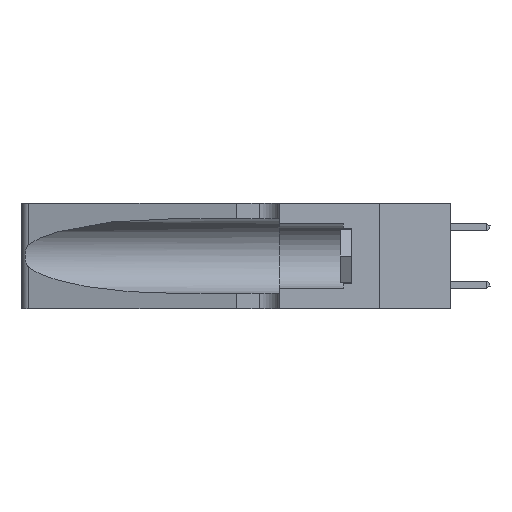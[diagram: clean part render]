
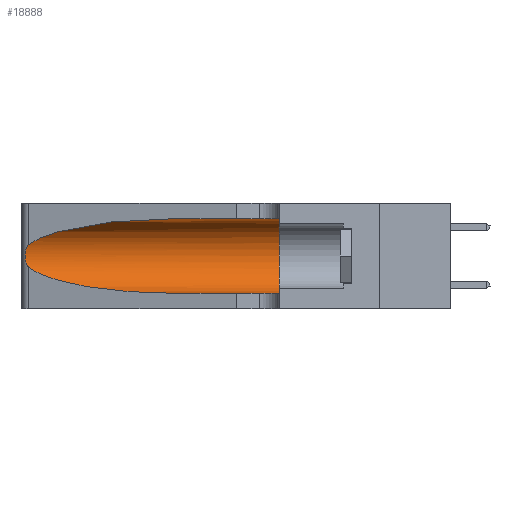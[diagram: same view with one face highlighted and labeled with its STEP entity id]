
A CAD part, left-side view. The second image highlights one B-rep face of the part: STEP entity #18888.
In plain terms, the highlighted cylindrical face has radius 3.308 mm (diameter 6.617 mm), a partial arc.
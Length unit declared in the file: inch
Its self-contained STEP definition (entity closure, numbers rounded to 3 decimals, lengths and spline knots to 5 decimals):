
#78 = CARTESIAN_POINT ( 'NONE',  ( 0.1305, 1.61858, 0.185 ) ) ;
#331 = AXIS2_PLACEMENT_3D ( 'NONE', #78, #10808, #15118 ) ;
#923 = VERTEX_POINT ( 'NONE', #23776 ) ;
#1726 = LINE ( 'NONE', #21640, #12320 ) ;
#1772 = CARTESIAN_POINT ( 'NONE',  ( 0.1305, 0.72297, 0.31525 ) ) ;
#1822 = EDGE_CURVE ( 'NONE', #23802, #9129, #22448, .T. ) ;
#2051 = CARTESIAN_POINT ( 'NONE',  ( 0.25856, 1.23593, 0.16098 ) ) ;
#2554 = CARTESIAN_POINT ( 'NONE',  ( 0.1305, 0.72297, 0.31525 ) ) ;
#3502 = ORIENTED_EDGE ( 'NONE', *, *, #5940, .T. ) ;
#3691 = CARTESIAN_POINT ( 'NONE',  ( 0.25487, 1.22718, 0.14631 ) ) ;
#4161 = CARTESIAN_POINT ( 'NONE',  ( 0.25639, 1.23186, 0.15144 ) ) ;
#5436 = CARTESIAN_POINT ( 'NONE',  ( 0.2373, 1.15595, 0.08982 ) ) ;
#5483 = LINE ( 'NONE', #10840, #10451 ) ;
#5678 = CIRCLE ( 'NONE', #11057, 0.13025 ) ;
#5940 = EDGE_CURVE ( 'NONE', #923, #23802, #12637, .T. ) ;
#6181 = VERTEX_POINT ( 'NONE', #7060 ) ;
#6287 = EDGE_CURVE ( 'NONE', #13009, #6181, #5678, .T. ) ;
#6307 = CARTESIAN_POINT ( 'NONE',  ( 0.25487, 1.22718, 0.14631 ) ) ;
#7060 = CARTESIAN_POINT ( 'NONE',  ( 0.1305, 0.35, 0.05475 ) ) ;
#8197 = CARTESIAN_POINT ( 'NONE',  ( 0.2373, 1.15595, 0.28018 ) ) ;
#8360 = CARTESIAN_POINT ( 'NONE',  ( 0.25639, 1.23184, 0.21858 ) ) ;
#8706 = FACE_OUTER_BOUND ( 'NONE', #13046, .T. ) ;
#9129 = VERTEX_POINT ( 'NONE', #16819 ) ;
#9145 = ORIENTED_EDGE ( 'NONE', *, *, #1822, .T. ) ;
#9790 = CARTESIAN_POINT ( 'NONE',  ( 0.25487, 1.22718, 0.14631 ) ) ;
#10451 = VECTOR ( 'NONE', #12997, 39.37008 ) ;
#10462 = CARTESIAN_POINT ( 'NONE',  ( 0.25854, 1.2359, 0.20912 ) ) ;
#10583 =( BOUNDED_CURVE ( )  B_SPLINE_CURVE ( 3, ( #1772, #20852, #8197, #22942 ),
 .UNSPECIFIED., .F., .F. ) 
 B_SPLINE_CURVE_WITH_KNOTS ( ( 4, 4 ),
 ( 1.5708, 2.84003 ),
 .UNSPECIFIED. ) 
 CURVE ( )  GEOMETRIC_REPRESENTATION_ITEM ( )  RATIONAL_B_SPLINE_CURVE ( ( 1., 0.87, 0.87, 1. ) ) 
 REPRESENTATION_ITEM ( '' )  );
#10808 = DIRECTION ( 'NONE',  ( 0., -1., 0. ) ) ;
#10840 = CARTESIAN_POINT ( 'NONE',  ( 0.1305, 1.61858, 0.05475 ) ) ;
#11057 = AXIS2_PLACEMENT_3D ( 'NONE', #24269, #11652, #26389 ) ;
#11652 = DIRECTION ( 'NONE',  ( 0., 1., 0. ) ) ;
#12277 = VERTEX_POINT ( 'NONE', #2554 ) ;
#12320 = VECTOR ( 'NONE', #23739, 39.37008 ) ;
#12603 = CARTESIAN_POINT ( 'NONE',  ( 0.26075, 1.23896, 0.19203 ) ) ;
#12637 = B_SPLINE_CURVE_WITH_KNOTS ( 'NONE', 3,
 ( #18894, #21031, #8360, #23122, #10462, #25224, #12603, #27333, #14761, #2051, #16870, #4161, #18993, #6307 ),
 .UNSPECIFIED., .F., .F.,
 ( 4, 2, 2, 2, 2, 2, 4 ),
 ( 0., 0.00027, 0.00053, 0.00107, 0.0016, 0.00187, 0.00214 ),
 .UNSPECIFIED. ) ;
#12997 = DIRECTION ( 'NONE',  ( 0., -1., 0. ) ) ;
#13009 = VERTEX_POINT ( 'NONE', #21774 ) ;
#13046 = EDGE_LOOP ( 'NONE', ( #14138, #3502, #9145, #26640, #16120, #22371 ) ) ;
#14138 = ORIENTED_EDGE ( 'NONE', *, *, #15998, .T. ) ;
#14761 = CARTESIAN_POINT ( 'NONE',  ( 0.26017, 1.23833, 0.17102 ) ) ;
#15118 = DIRECTION ( 'NONE',  ( 0., 0., -1. ) ) ;
#15998 = EDGE_CURVE ( 'NONE', #12277, #923, #10583, .T. ) ;
#16120 = ORIENTED_EDGE ( 'NONE', *, *, #6287, .F. ) ;
#16819 = CARTESIAN_POINT ( 'NONE',  ( 0.1305, 0.72297, 0.05475 ) ) ;
#16870 = CARTESIAN_POINT ( 'NONE',  ( 0.25789, 1.23486, 0.15765 ) ) ;
#18888 = ADVANCED_FACE ( 'NONE', ( #8706 ), #24859, .F. ) ;
#18894 = CARTESIAN_POINT ( 'NONE',  ( 0.25487, 1.22718, 0.22369 ) ) ;
#18942 = EDGE_CURVE ( 'NONE', #12277, #13009, #1726, .T. ) ;
#18993 = CARTESIAN_POINT ( 'NONE',  ( 0.25555, 1.22993, 0.14849 ) ) ;
#20346 = CARTESIAN_POINT ( 'NONE',  ( 0.18966, 0.96281, 0.05475 ) ) ;
#20852 = CARTESIAN_POINT ( 'NONE',  ( 0.18966, 0.96281, 0.31525 ) ) ;
#21031 = CARTESIAN_POINT ( 'NONE',  ( 0.25555, 1.22994, 0.2215 ) ) ;
#21640 = CARTESIAN_POINT ( 'NONE',  ( 0.1305, 1.61858, 0.31525 ) ) ;
#21774 = CARTESIAN_POINT ( 'NONE',  ( 0.1305, 0.35, 0.31525 ) ) ;
#22371 = ORIENTED_EDGE ( 'NONE', *, *, #18942, .F. ) ;
#22448 =( BOUNDED_CURVE ( )  B_SPLINE_CURVE ( 3, ( #9790, #5436, #20346, #24545 ),
 .UNSPECIFIED., .F., .T. ) 
 B_SPLINE_CURVE_WITH_KNOTS ( ( 4, 4 ),
 ( 3.44316, 4.71239 ),
 .UNSPECIFIED. ) 
 CURVE ( )  GEOMETRIC_REPRESENTATION_ITEM ( )  RATIONAL_B_SPLINE_CURVE ( ( 1., 0.87, 0.87, 1. ) ) 
 REPRESENTATION_ITEM ( '' )  );
#22942 = CARTESIAN_POINT ( 'NONE',  ( 0.25487, 1.22718, 0.22369 ) ) ;
#23122 = CARTESIAN_POINT ( 'NONE',  ( 0.25787, 1.23484, 0.2124 ) ) ;
#23346 = EDGE_CURVE ( 'NONE', #9129, #6181, #5483, .T. ) ;
#23739 = DIRECTION ( 'NONE',  ( 0., -1., 0. ) ) ;
#23776 = CARTESIAN_POINT ( 'NONE',  ( 0.25487, 1.22718, 0.22369 ) ) ;
#23802 = VERTEX_POINT ( 'NONE', #3691 ) ;
#24269 = CARTESIAN_POINT ( 'NONE',  ( 0.1305, 0.35, 0.185 ) ) ;
#24545 = CARTESIAN_POINT ( 'NONE',  ( 0.1305, 0.72297, 0.05475 ) ) ;
#24859 = CYLINDRICAL_SURFACE ( 'NONE', #331, 0.13025 ) ;
#25224 = CARTESIAN_POINT ( 'NONE',  ( 0.26018, 1.23835, 0.19895 ) ) ;
#26389 = DIRECTION ( 'NONE',  ( 0., 0., 1. ) ) ;
#26640 = ORIENTED_EDGE ( 'NONE', *, *, #23346, .T. ) ;
#27333 = CARTESIAN_POINT ( 'NONE',  ( 0.26075, 1.23896, 0.178 ) ) ;
